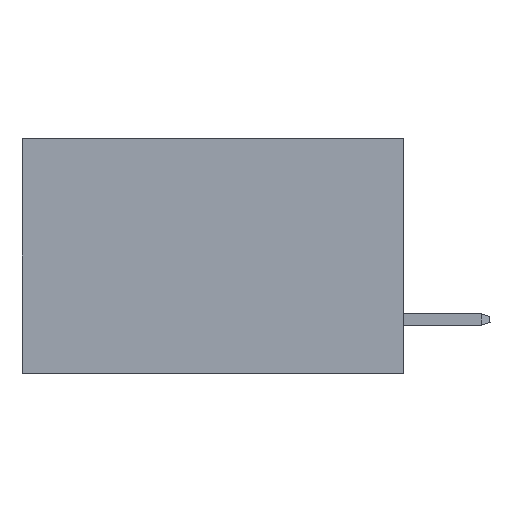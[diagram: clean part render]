
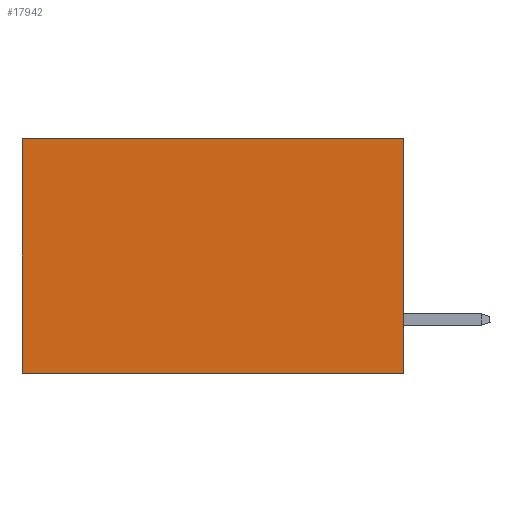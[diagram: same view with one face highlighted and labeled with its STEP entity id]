
A CAD part, left-side view. The second image highlights one B-rep face of the part: STEP entity #17942.
In plain terms, the highlighted planar face has unit normal (-1, 0, 0).
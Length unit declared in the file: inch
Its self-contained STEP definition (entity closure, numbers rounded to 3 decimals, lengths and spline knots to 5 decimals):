
#403 = VERTEX_POINT ( 'NONE', #8578 ) ;
#823 = LINE ( 'NONE', #7265, #18820 ) ;
#1619 = VECTOR ( 'NONE', #14063, 39.37008 ) ;
#1800 = EDGE_CURVE ( 'NONE', #15135, #16646, #2661, .T. ) ;
#2184 = ORIENTED_EDGE ( 'NONE', *, *, #1800, .T. ) ;
#2274 = EDGE_CURVE ( 'NONE', #4306, #403, #7485, .T. ) ;
#2661 = LINE ( 'NONE', #5606, #1619 ) ;
#3296 = CARTESIAN_POINT ( 'NONE',  ( 0.2875, 0.6, -0.37 ) ) ;
#3301 = PLANE ( 'NONE',  #16786 ) ;
#4109 = DIRECTION ( 'NONE',  ( 0., 0., -1. ) ) ;
#4306 = VERTEX_POINT ( 'NONE', #12662 ) ;
#5000 = ORIENTED_EDGE ( 'NONE', *, *, #2274, .F. ) ;
#5606 = CARTESIAN_POINT ( 'NONE',  ( 0.2875, 0.6, 0. ) ) ;
#6190 = LINE ( 'NONE', #15903, #19832 ) ;
#7192 = EDGE_CURVE ( 'NONE', #4306, #15135, #823, .T. ) ;
#7265 = CARTESIAN_POINT ( 'NONE',  ( 0.2875, 0., 0. ) ) ;
#7485 = LINE ( 'NONE', #10442, #19252 ) ;
#7778 = DIRECTION ( 'NONE',  ( 0., 1., 0. ) ) ;
#8381 = EDGE_CURVE ( 'NONE', #403, #16646, #6190, .T. ) ;
#8578 = CARTESIAN_POINT ( 'NONE',  ( 0.2875, 0., -0.37 ) ) ;
#9741 = DIRECTION ( 'NONE',  ( 1., 0., 0. ) ) ;
#10442 = CARTESIAN_POINT ( 'NONE',  ( 0.2875, 0., 0. ) ) ;
#11577 = ORIENTED_EDGE ( 'NONE', *, *, #7192, .T. ) ;
#11632 = DIRECTION ( 'NONE',  ( 0., 0., -1. ) ) ;
#12131 = DIRECTION ( 'NONE',  ( 0., 1., 0. ) ) ;
#12662 = CARTESIAN_POINT ( 'NONE',  ( 0.2875, 0., 0. ) ) ;
#12786 = EDGE_LOOP ( 'NONE', ( #2184, #18810, #5000, #11577 ) ) ;
#13327 = FACE_OUTER_BOUND ( 'NONE', #12786, .T. ) ;
#14063 = DIRECTION ( 'NONE',  ( 0., 0., -1. ) ) ;
#14905 = CARTESIAN_POINT ( 'NONE',  ( 0.2875, 0., 0. ) ) ;
#15135 = VERTEX_POINT ( 'NONE', #15659 ) ;
#15659 = CARTESIAN_POINT ( 'NONE',  ( 0.2875, 0.6, 0. ) ) ;
#15903 = CARTESIAN_POINT ( 'NONE',  ( 0.2875, 0., -0.37 ) ) ;
#16646 = VERTEX_POINT ( 'NONE', #3296 ) ;
#16786 = AXIS2_PLACEMENT_3D ( 'NONE', #14905, #9741, #11632 ) ;
#17942 = ADVANCED_FACE ( 'NONE', ( #13327 ), #3301, .F. ) ;
#18810 = ORIENTED_EDGE ( 'NONE', *, *, #8381, .F. ) ;
#18820 = VECTOR ( 'NONE', #12131, 39.37008 ) ;
#19252 = VECTOR ( 'NONE', #4109, 39.37008 ) ;
#19832 = VECTOR ( 'NONE', #7778, 39.37008 ) ;
